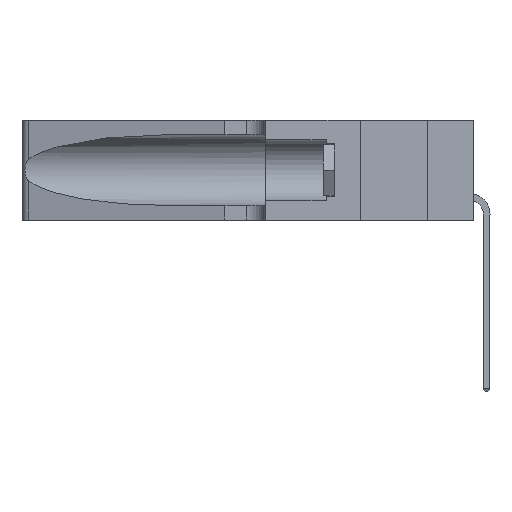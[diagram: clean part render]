
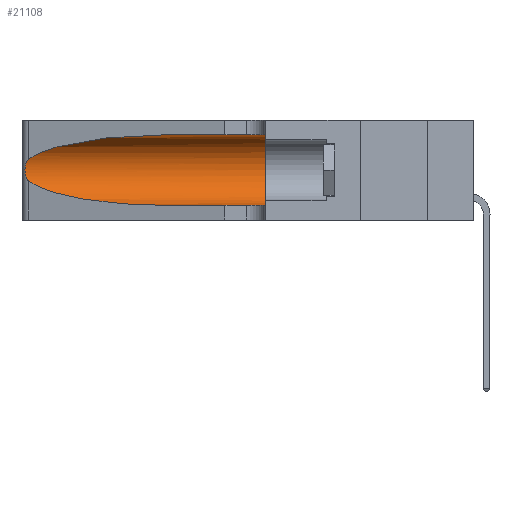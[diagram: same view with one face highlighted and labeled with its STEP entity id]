
A CAD part, left-side view. The second image highlights one B-rep face of the part: STEP entity #21108.
In plain terms, the highlighted cylindrical face has radius 3.308 mm (diameter 6.617 mm), a partial arc.
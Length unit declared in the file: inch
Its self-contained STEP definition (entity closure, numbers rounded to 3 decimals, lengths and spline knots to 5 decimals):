
#9 = CARTESIAN_POINT ( 'NONE',  ( 0.1305, 1.61858, 0.05475 ) ) ;
#383 = FACE_OUTER_BOUND ( 'NONE', #16481, .T. ) ;
#754 = CARTESIAN_POINT ( 'NONE',  ( 0.26017, 1.23833, 0.17102 ) ) ;
#836 = CARTESIAN_POINT ( 'NONE',  ( 0.25555, 1.22994, 0.2215 ) ) ;
#950 = LINE ( 'NONE', #9, #15570 ) ;
#1005 = VERTEX_POINT ( 'NONE', #14918 ) ;
#1754 = B_SPLINE_CURVE_WITH_KNOTS ( 'NONE', 3,
 ( #15588, #836, #18882, #12342, #10717, #8832, #7460, #12499, #754, #15861, #2475, #5637, #14096, #4085 ),
 .UNSPECIFIED., .F., .F.,
 ( 4, 2, 2, 2, 2, 2, 4 ),
 ( 0., 0.00027, 0.00053, 0.00107, 0.0016, 0.00187, 0.00214 ),
 .UNSPECIFIED. ) ;
#1858 = EDGE_CURVE ( 'NONE', #1005, #19718, #12738, .T. ) ;
#2035 = CARTESIAN_POINT ( 'NONE',  ( 0.25487, 1.22718, 0.22369 ) ) ;
#2475 = CARTESIAN_POINT ( 'NONE',  ( 0.25789, 1.23486, 0.15765 ) ) ;
#3096 = CARTESIAN_POINT ( 'NONE',  ( 0.1305, 0.35, 0.05475 ) ) ;
#3331 =( BOUNDED_CURVE ( )  B_SPLINE_CURVE ( 3, ( #3870, #12125, #3793, #5653 ),
 .UNSPECIFIED., .F., .F. ) 
 B_SPLINE_CURVE_WITH_KNOTS ( ( 4, 4 ),
 ( 1.5708, 2.84003 ),
 .UNSPECIFIED. ) 
 CURVE ( )  GEOMETRIC_REPRESENTATION_ITEM ( )  RATIONAL_B_SPLINE_CURVE ( ( 1., 0.87, 0.87, 1. ) ) 
 REPRESENTATION_ITEM ( '' )  );
#3788 = ORIENTED_EDGE ( 'NONE', *, *, #10799, .F. ) ;
#3793 = CARTESIAN_POINT ( 'NONE',  ( 0.2373, 1.15595, 0.28018 ) ) ;
#3870 = CARTESIAN_POINT ( 'NONE',  ( 0.1305, 0.72297, 0.31525 ) ) ;
#4010 = VECTOR ( 'NONE', #13029, 39.37008 ) ;
#4085 = CARTESIAN_POINT ( 'NONE',  ( 0.25487, 1.22718, 0.14631 ) ) ;
#4186 = ORIENTED_EDGE ( 'NONE', *, *, #5034, .F. ) ;
#5034 = EDGE_CURVE ( 'NONE', #18476, #11133, #20221, .T. ) ;
#5637 = CARTESIAN_POINT ( 'NONE',  ( 0.25639, 1.23186, 0.15144 ) ) ;
#5653 = CARTESIAN_POINT ( 'NONE',  ( 0.25487, 1.22718, 0.22369 ) ) ;
#5764 = AXIS2_PLACEMENT_3D ( 'NONE', #12477, #9533, #19569 ) ;
#6401 = CARTESIAN_POINT ( 'NONE',  ( 0.1305, 1.61858, 0.31525 ) ) ;
#6407 = ORIENTED_EDGE ( 'NONE', *, *, #14010, .T. ) ;
#6969 = EDGE_CURVE ( 'NONE', #19718, #10806, #950, .T. ) ;
#7175 = ORIENTED_EDGE ( 'NONE', *, *, #1858, .T. ) ;
#7460 = CARTESIAN_POINT ( 'NONE',  ( 0.26075, 1.23896, 0.19203 ) ) ;
#7779 = CARTESIAN_POINT ( 'NONE',  ( 0.1305, 0.72297, 0.31525 ) ) ;
#8113 = CARTESIAN_POINT ( 'NONE',  ( 0.1305, 0.72297, 0.05475 ) ) ;
#8832 = CARTESIAN_POINT ( 'NONE',  ( 0.26018, 1.23835, 0.19895 ) ) ;
#8977 = EDGE_CURVE ( 'NONE', #18476, #18892, #3331, .T. ) ;
#9104 = AXIS2_PLACEMENT_3D ( 'NONE', #14823, #9800, #14889 ) ;
#9533 = DIRECTION ( 'NONE',  ( 0., -1., 0. ) ) ;
#9800 = DIRECTION ( 'NONE',  ( 0., 1., 0. ) ) ;
#10009 = CYLINDRICAL_SURFACE ( 'NONE', #5764, 0.13025 ) ;
#10717 = CARTESIAN_POINT ( 'NONE',  ( 0.25854, 1.2359, 0.20912 ) ) ;
#10799 = EDGE_CURVE ( 'NONE', #11133, #10806, #21143, .T. ) ;
#10806 = VERTEX_POINT ( 'NONE', #3096 ) ;
#11133 = VERTEX_POINT ( 'NONE', #14749 ) ;
#12125 = CARTESIAN_POINT ( 'NONE',  ( 0.18966, 0.96281, 0.31525 ) ) ;
#12342 = CARTESIAN_POINT ( 'NONE',  ( 0.25787, 1.23484, 0.2124 ) ) ;
#12477 = CARTESIAN_POINT ( 'NONE',  ( 0.1305, 1.61858, 0.185 ) ) ;
#12499 = CARTESIAN_POINT ( 'NONE',  ( 0.26075, 1.23896, 0.178 ) ) ;
#12611 = CARTESIAN_POINT ( 'NONE',  ( 0.2373, 1.15595, 0.08982 ) ) ;
#12738 =( BOUNDED_CURVE ( )  B_SPLINE_CURVE ( 3, ( #19501, #12611, #14298, #14528 ),
 .UNSPECIFIED., .F., .T. ) 
 B_SPLINE_CURVE_WITH_KNOTS ( ( 4, 4 ),
 ( 3.44316, 4.71239 ),
 .UNSPECIFIED. ) 
 CURVE ( )  GEOMETRIC_REPRESENTATION_ITEM ( )  RATIONAL_B_SPLINE_CURVE ( ( 1., 0.87, 0.87, 1. ) ) 
 REPRESENTATION_ITEM ( '' )  );
#13029 = DIRECTION ( 'NONE',  ( 0., -1., 0. ) ) ;
#14010 = EDGE_CURVE ( 'NONE', #18892, #1005, #1754, .T. ) ;
#14096 = CARTESIAN_POINT ( 'NONE',  ( 0.25555, 1.22993, 0.14849 ) ) ;
#14298 = CARTESIAN_POINT ( 'NONE',  ( 0.18966, 0.96281, 0.05475 ) ) ;
#14528 = CARTESIAN_POINT ( 'NONE',  ( 0.1305, 0.72297, 0.05475 ) ) ;
#14694 = ORIENTED_EDGE ( 'NONE', *, *, #6969, .T. ) ;
#14749 = CARTESIAN_POINT ( 'NONE',  ( 0.1305, 0.35, 0.31525 ) ) ;
#14823 = CARTESIAN_POINT ( 'NONE',  ( 0.1305, 0.35, 0.185 ) ) ;
#14889 = DIRECTION ( 'NONE',  ( 0., 0., 1. ) ) ;
#14918 = CARTESIAN_POINT ( 'NONE',  ( 0.25487, 1.22718, 0.14631 ) ) ;
#15570 = VECTOR ( 'NONE', #18496, 39.37008 ) ;
#15588 = CARTESIAN_POINT ( 'NONE',  ( 0.25487, 1.22718, 0.22369 ) ) ;
#15861 = CARTESIAN_POINT ( 'NONE',  ( 0.25856, 1.23593, 0.16098 ) ) ;
#16481 = EDGE_LOOP ( 'NONE', ( #17139, #6407, #7175, #14694, #3788, #4186 ) ) ;
#17139 = ORIENTED_EDGE ( 'NONE', *, *, #8977, .T. ) ;
#18476 = VERTEX_POINT ( 'NONE', #7779 ) ;
#18496 = DIRECTION ( 'NONE',  ( 0., -1., 0. ) ) ;
#18882 = CARTESIAN_POINT ( 'NONE',  ( 0.25639, 1.23184, 0.21858 ) ) ;
#18892 = VERTEX_POINT ( 'NONE', #2035 ) ;
#19501 = CARTESIAN_POINT ( 'NONE',  ( 0.25487, 1.22718, 0.14631 ) ) ;
#19569 = DIRECTION ( 'NONE',  ( 0., 0., -1. ) ) ;
#19718 = VERTEX_POINT ( 'NONE', #8113 ) ;
#20221 = LINE ( 'NONE', #6401, #4010 ) ;
#21108 = ADVANCED_FACE ( 'NONE', ( #383 ), #10009, .F. ) ;
#21143 = CIRCLE ( 'NONE', #9104, 0.13025 ) ;
